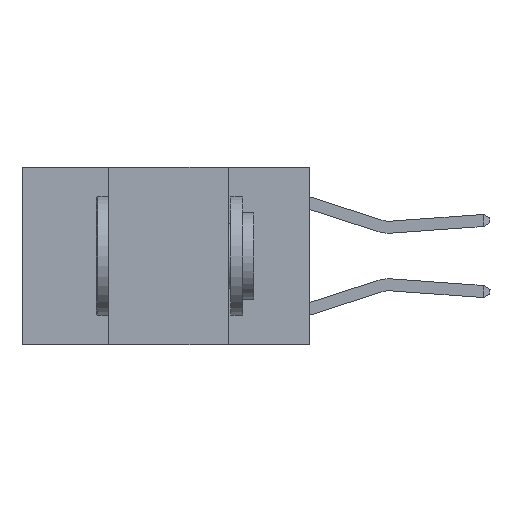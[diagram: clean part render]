
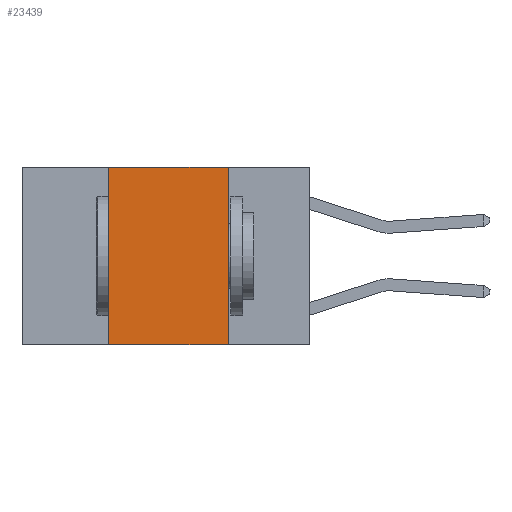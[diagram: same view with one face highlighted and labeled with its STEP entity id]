
A CAD part, left-side view. The second image highlights one B-rep face of the part: STEP entity #23439.
In plain terms, the highlighted planar face has unit normal (-1, 0, 0).
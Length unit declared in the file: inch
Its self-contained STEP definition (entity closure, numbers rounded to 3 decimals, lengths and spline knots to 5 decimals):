
#189 = EDGE_CURVE ( 'NONE', #11635, #17026, #9934, .T. ) ;
#921 = VECTOR ( 'NONE', #18460, 39.37008 ) ;
#1073 = EDGE_CURVE ( 'NONE', #17026, #2713, #1423, .T. ) ;
#1423 = LINE ( 'NONE', #2818, #22736 ) ;
#2521 = DIRECTION ( 'NONE',  ( 0., -1., 0. ) ) ;
#2713 = VERTEX_POINT ( 'NONE', #4364 ) ;
#2818 = CARTESIAN_POINT ( 'NONE',  ( 0., 0.6, 0. ) ) ;
#2873 = VECTOR ( 'NONE', #18188, 39.37008 ) ;
#3904 = EDGE_CURVE ( 'NONE', #11635, #15689, #13918, .T. ) ;
#4364 = CARTESIAN_POINT ( 'NONE',  ( 0., 0.17, 0. ) ) ;
#4672 = ORIENTED_EDGE ( 'NONE', *, *, #3904, .T. ) ;
#9502 = CARTESIAN_POINT ( 'NONE',  ( 0., 0.42, 0. ) ) ;
#9934 = LINE ( 'NONE', #21377, #15441 ) ;
#11419 = CARTESIAN_POINT ( 'NONE',  ( 0., 0.42, -0.37 ) ) ;
#11635 = VERTEX_POINT ( 'NONE', #11419 ) ;
#11894 = DIRECTION ( 'NONE',  ( 1., 0., 0. ) ) ;
#13824 = EDGE_LOOP ( 'NONE', ( #19162, #24620, #25927, #4672 ) ) ;
#13902 = LINE ( 'NONE', #22318, #2873 ) ;
#13918 = LINE ( 'NONE', #26632, #921 ) ;
#15441 = VECTOR ( 'NONE', #21437, 39.37008 ) ;
#15689 = VERTEX_POINT ( 'NONE', #19064 ) ;
#17026 = VERTEX_POINT ( 'NONE', #9502 ) ;
#18188 = DIRECTION ( 'NONE',  ( 0., 0., -1. ) ) ;
#18460 = DIRECTION ( 'NONE',  ( 0., -1., 0. ) ) ;
#18557 = AXIS2_PLACEMENT_3D ( 'NONE', #24184, #11894, #26253 ) ;
#19064 = CARTESIAN_POINT ( 'NONE',  ( 0., 0.17, -0.37 ) ) ;
#19162 = ORIENTED_EDGE ( 'NONE', *, *, #19780, .F. ) ;
#19780 = EDGE_CURVE ( 'NONE', #2713, #15689, #13902, .T. ) ;
#19957 = PLANE ( 'NONE',  #18557 ) ;
#21377 = CARTESIAN_POINT ( 'NONE',  ( 0., 0.42, 0. ) ) ;
#21437 = DIRECTION ( 'NONE',  ( 0., 0., 1. ) ) ;
#22318 = CARTESIAN_POINT ( 'NONE',  ( 0., 0.17, 0. ) ) ;
#22736 = VECTOR ( 'NONE', #2521, 39.37008 ) ;
#23439 = ADVANCED_FACE ( 'NONE', ( #25249 ), #19957, .F. ) ;
#24184 = CARTESIAN_POINT ( 'NONE',  ( 0., 0.6, 0. ) ) ;
#24620 = ORIENTED_EDGE ( 'NONE', *, *, #1073, .F. ) ;
#25249 = FACE_OUTER_BOUND ( 'NONE', #13824, .T. ) ;
#25927 = ORIENTED_EDGE ( 'NONE', *, *, #189, .F. ) ;
#26253 = DIRECTION ( 'NONE',  ( 0., 0., -1. ) ) ;
#26632 = CARTESIAN_POINT ( 'NONE',  ( 0., 0.6, -0.37 ) ) ;
